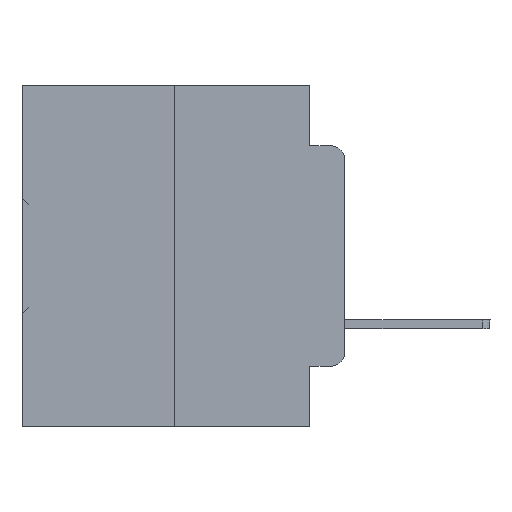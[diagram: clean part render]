
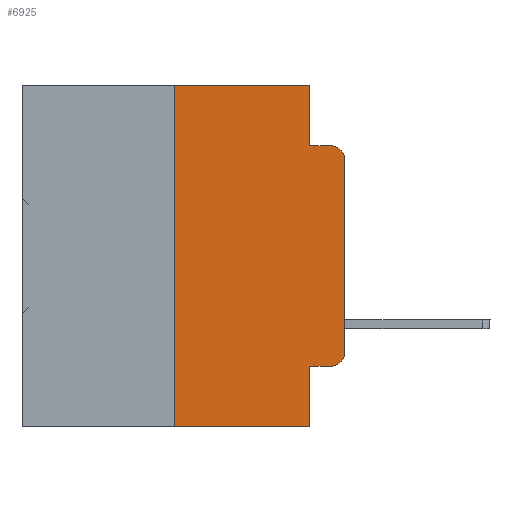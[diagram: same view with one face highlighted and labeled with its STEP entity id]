
A CAD part, left-side view. The second image highlights one B-rep face of the part: STEP entity #6925.
In plain terms, the highlighted planar face has unit normal (-1, 0, 0).
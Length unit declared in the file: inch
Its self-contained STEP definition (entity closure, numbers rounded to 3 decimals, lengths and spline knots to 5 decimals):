
#173 = AXIS2_PLACEMENT_3D ( 'NONE', #4027, #26258, #1308 ) ;
#478 = CARTESIAN_POINT ( 'NONE',  ( 0., 0., -0.3915 ) ) ;
#995 = ORIENTED_EDGE ( 'NONE', *, *, #14042, .T. ) ;
#1199 = ORIENTED_EDGE ( 'NONE', *, *, #15317, .T. ) ;
#1264 = VERTEX_POINT ( 'NONE', #14178 ) ;
#1308 = DIRECTION ( 'NONE',  ( 0., 0., -1. ) ) ;
#1323 = ORIENTED_EDGE ( 'NONE', *, *, #22719, .T. ) ;
#1781 = CARTESIAN_POINT ( 'NONE',  ( 0., 0.02, -0.0885 ) ) ;
#2002 = DIRECTION ( 'NONE',  ( 0., 0., -1. ) ) ;
#2351 = CARTESIAN_POINT ( 'NONE',  ( 0., 0.051, 0. ) ) ;
#3365 = LINE ( 'NONE', #22529, #30025 ) ;
#4027 = CARTESIAN_POINT ( 'NONE',  ( 0., 0.473, 0. ) ) ;
#4825 = CARTESIAN_POINT ( 'NONE',  ( 0., 0.25, 0. ) ) ;
#5075 = DIRECTION ( 'NONE',  ( 0., 0., 1. ) ) ;
#5180 = LINE ( 'NONE', #24672, #16337 ) ;
#5266 = EDGE_CURVE ( 'NONE', #15309, #27697, #9701, .T. ) ;
#5324 = ORIENTED_EDGE ( 'NONE', *, *, #22731, .F. ) ;
#5480 = VECTOR ( 'NONE', #2002, 39.37008 ) ;
#6925 = ADVANCED_FACE ( 'NONE', ( #10236 ), #32440, .F. ) ;
#7494 = CIRCLE ( 'NONE', #20894, 0.02 ) ;
#7853 = EDGE_LOOP ( 'NONE', ( #1199, #1323, #25813, #19685, #15071, #5324, #995, #26667, #16677, #30268 ) ) ;
#8366 = CARTESIAN_POINT ( 'NONE',  ( 0., 0., 0. ) ) ;
#8978 = EDGE_CURVE ( 'NONE', #27697, #10903, #15425, .T. ) ;
#9214 = DIRECTION ( 'NONE',  ( -1., 0., 0. ) ) ;
#9522 = DIRECTION ( 'NONE',  ( 0., -1., 0. ) ) ;
#9701 = LINE ( 'NONE', #25715, #23311 ) ;
#9747 = DIRECTION ( 'NONE',  ( 0., 0., -1. ) ) ;
#9896 = CARTESIAN_POINT ( 'NONE',  ( 0., 0.25, -0.5 ) ) ;
#9947 = EDGE_CURVE ( 'NONE', #20927, #34100, #15851, .T. ) ;
#10084 = VECTOR ( 'NONE', #23464, 39.37008 ) ;
#10236 = FACE_OUTER_BOUND ( 'NONE', #7853, .T. ) ;
#10903 = VERTEX_POINT ( 'NONE', #25709 ) ;
#11387 = DIRECTION ( 'NONE',  ( 0., -1., 0. ) ) ;
#11926 = LINE ( 'NONE', #20325, #13072 ) ;
#12639 = VERTEX_POINT ( 'NONE', #1781 ) ;
#13072 = VECTOR ( 'NONE', #28857, 39.37008 ) ;
#14042 = EDGE_CURVE ( 'NONE', #14735, #34100, #3365, .T. ) ;
#14178 = CARTESIAN_POINT ( 'NONE',  ( 0., 0.02, -0.4115 ) ) ;
#14180 = LINE ( 'NONE', #8366, #33522 ) ;
#14735 = VERTEX_POINT ( 'NONE', #9896 ) ;
#14803 = CARTESIAN_POINT ( 'NONE',  ( 0., 0.051, -0.4115 ) ) ;
#15071 = ORIENTED_EDGE ( 'NONE', *, *, #5266, .F. ) ;
#15309 = VERTEX_POINT ( 'NONE', #16560 ) ;
#15317 = EDGE_CURVE ( 'NONE', #35304, #19534, #14180, .T. ) ;
#15425 = LINE ( 'NONE', #34372, #10084 ) ;
#15851 = LINE ( 'NONE', #2351, #5480 ) ;
#16337 = VECTOR ( 'NONE', #11387, 39.37008 ) ;
#16560 = CARTESIAN_POINT ( 'NONE',  ( 0., 0.25, 0. ) ) ;
#16677 = ORIENTED_EDGE ( 'NONE', *, *, #22935, .T. ) ;
#16896 = CIRCLE ( 'NONE', #33193, 0.02 ) ;
#18132 = LINE ( 'NONE', #4825, #21570 ) ;
#19534 = VERTEX_POINT ( 'NONE', #22825 ) ;
#19685 = ORIENTED_EDGE ( 'NONE', *, *, #8978, .F. ) ;
#20325 = CARTESIAN_POINT ( 'NONE',  ( 0., 0.051, -0.0885 ) ) ;
#20894 = AXIS2_PLACEMENT_3D ( 'NONE', #31387, #9214, #9747 ) ;
#20927 = VERTEX_POINT ( 'NONE', #14803 ) ;
#21570 = VECTOR ( 'NONE', #26693, 39.37008 ) ;
#22529 = CARTESIAN_POINT ( 'NONE',  ( 0., 0.473, -0.5 ) ) ;
#22719 = EDGE_CURVE ( 'NONE', #19534, #12639, #16896, .T. ) ;
#22731 = EDGE_CURVE ( 'NONE', #14735, #15309, #18132, .T. ) ;
#22755 = CARTESIAN_POINT ( 'NONE',  ( 0., 0.051, -0.5 ) ) ;
#22825 = CARTESIAN_POINT ( 'NONE',  ( 0., 0., -0.1085 ) ) ;
#22935 = EDGE_CURVE ( 'NONE', #20927, #1264, #5180, .T. ) ;
#23311 = VECTOR ( 'NONE', #9522, 39.37008 ) ;
#23464 = DIRECTION ( 'NONE',  ( 0., 0., -1. ) ) ;
#23785 = DIRECTION ( 'NONE',  ( -1., 0., 0. ) ) ;
#24672 = CARTESIAN_POINT ( 'NONE',  ( 0., 0.051, -0.4115 ) ) ;
#25709 = CARTESIAN_POINT ( 'NONE',  ( 0., 0.051, -0.0885 ) ) ;
#25715 = CARTESIAN_POINT ( 'NONE',  ( 0., 0.473, 0. ) ) ;
#25813 = ORIENTED_EDGE ( 'NONE', *, *, #34386, .F. ) ;
#26258 = DIRECTION ( 'NONE',  ( 1., 0., 0. ) ) ;
#26667 = ORIENTED_EDGE ( 'NONE', *, *, #9947, .F. ) ;
#26693 = DIRECTION ( 'NONE',  ( 0., 0., 1. ) ) ;
#26783 = EDGE_CURVE ( 'NONE', #1264, #35304, #7494, .T. ) ;
#27697 = VERTEX_POINT ( 'NONE', #33867 ) ;
#28857 = DIRECTION ( 'NONE',  ( 0., -1., 0. ) ) ;
#30025 = VECTOR ( 'NONE', #33248, 39.37008 ) ;
#30268 = ORIENTED_EDGE ( 'NONE', *, *, #26783, .T. ) ;
#31387 = CARTESIAN_POINT ( 'NONE',  ( 0., 0.02, -0.3915 ) ) ;
#31972 = CARTESIAN_POINT ( 'NONE',  ( 0., 0.02, -0.1085 ) ) ;
#32440 = PLANE ( 'NONE',  #173 ) ;
#33193 = AXIS2_PLACEMENT_3D ( 'NONE', #31972, #23785, #35424 ) ;
#33248 = DIRECTION ( 'NONE',  ( 0., -1., 0. ) ) ;
#33522 = VECTOR ( 'NONE', #5075, 39.37008 ) ;
#33867 = CARTESIAN_POINT ( 'NONE',  ( 0., 0.051, 0. ) ) ;
#34100 = VERTEX_POINT ( 'NONE', #22755 ) ;
#34372 = CARTESIAN_POINT ( 'NONE',  ( 0., 0.051, 0. ) ) ;
#34386 = EDGE_CURVE ( 'NONE', #10903, #12639, #11926, .T. ) ;
#35304 = VERTEX_POINT ( 'NONE', #478 ) ;
#35424 = DIRECTION ( 'NONE',  ( 0., 0., -1. ) ) ;
